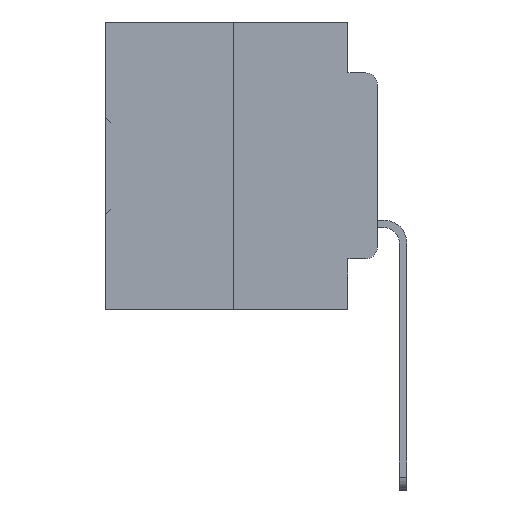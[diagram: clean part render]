
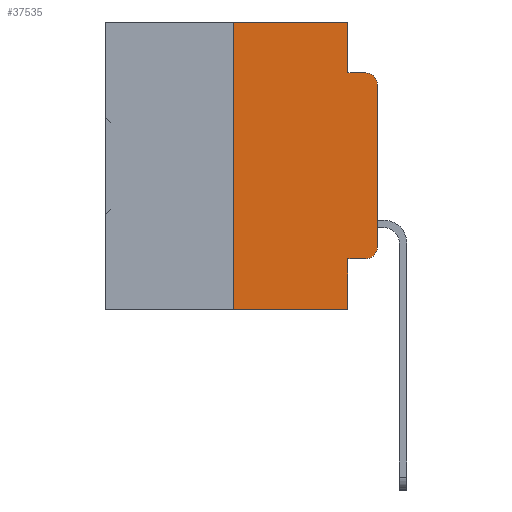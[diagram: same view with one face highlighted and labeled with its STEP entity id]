
A CAD part, left-side view. The second image highlights one B-rep face of the part: STEP entity #37535.
In plain terms, the highlighted planar face has unit normal (-1, 0, 0).
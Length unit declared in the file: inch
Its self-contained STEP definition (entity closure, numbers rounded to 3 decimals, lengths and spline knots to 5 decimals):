
#149 = EDGE_CURVE ( 'NONE', #15255, #26655, #14297, .T. ) ;
#2393 = DIRECTION ( 'NONE',  ( -1., 0., 0. ) ) ;
#2667 = CIRCLE ( 'NONE', #27119, 0.02 ) ;
#3807 = AXIS2_PLACEMENT_3D ( 'NONE', #12877, #33331, #15895 ) ;
#4180 = CARTESIAN_POINT ( 'NONE',  ( 0., 0.051, 0. ) ) ;
#6223 = CARTESIAN_POINT ( 'NONE',  ( 0., 0.051, -0.0885 ) ) ;
#8025 = CARTESIAN_POINT ( 'NONE',  ( 0., 0.25, 0. ) ) ;
#8068 = CARTESIAN_POINT ( 'NONE',  ( 0., 0.02, -0.4115 ) ) ;
#8298 = EDGE_CURVE ( 'NONE', #8849, #34563, #30293, .T. ) ;
#8849 = VERTEX_POINT ( 'NONE', #18146 ) ;
#9312 = LINE ( 'NONE', #22283, #16289 ) ;
#9317 = CARTESIAN_POINT ( 'NONE',  ( 0., 0.25, 0. ) ) ;
#9435 = CARTESIAN_POINT ( 'NONE',  ( 0., 0.02, -0.1085 ) ) ;
#9845 = CARTESIAN_POINT ( 'NONE',  ( 0., 0.02, -0.0885 ) ) ;
#9890 = CARTESIAN_POINT ( 'NONE',  ( 0., 0.051, 0. ) ) ;
#10317 = CARTESIAN_POINT ( 'NONE',  ( 0., 0.051, -0.5 ) ) ;
#11504 = DIRECTION ( 'NONE',  ( 0., -1., 0. ) ) ;
#12415 = DIRECTION ( 'NONE',  ( 0., 0., -1. ) ) ;
#12753 = PLANE ( 'NONE',  #3807 ) ;
#12877 = CARTESIAN_POINT ( 'NONE',  ( 0., 0.473, 0. ) ) ;
#13084 = VECTOR ( 'NONE', #24764, 39.37008 ) ;
#13214 = VERTEX_POINT ( 'NONE', #25533 ) ;
#13695 = EDGE_CURVE ( 'NONE', #14173, #29882, #20017, .T. ) ;
#14173 = VERTEX_POINT ( 'NONE', #8025 ) ;
#14297 = LINE ( 'NONE', #6223, #36649 ) ;
#14536 = ORIENTED_EDGE ( 'NONE', *, *, #15322, .T. ) ;
#14876 = VECTOR ( 'NONE', #24583, 39.37008 ) ;
#15255 = VERTEX_POINT ( 'NONE', #24947 ) ;
#15322 = EDGE_CURVE ( 'NONE', #20189, #30032, #9312, .T. ) ;
#15479 = CARTESIAN_POINT ( 'NONE',  ( 0., 0.051, 0. ) ) ;
#15895 = DIRECTION ( 'NONE',  ( 0., 0., -1. ) ) ;
#15964 = ORIENTED_EDGE ( 'NONE', *, *, #31698, .T. ) ;
#16280 = EDGE_CURVE ( 'NONE', #13214, #14173, #26963, .T. ) ;
#16289 = VECTOR ( 'NONE', #16528, 39.37008 ) ;
#16528 = DIRECTION ( 'NONE',  ( 0., 0., 1. ) ) ;
#16646 = CARTESIAN_POINT ( 'NONE',  ( 0., 0., -0.1085 ) ) ;
#16747 = ORIENTED_EDGE ( 'NONE', *, *, #149, .F. ) ;
#16749 = LINE ( 'NONE', #9890, #14876 ) ;
#17226 = ORIENTED_EDGE ( 'NONE', *, *, #26038, .F. ) ;
#17313 = CARTESIAN_POINT ( 'NONE',  ( 0., 0.051, -0.4115 ) ) ;
#18146 = CARTESIAN_POINT ( 'NONE',  ( 0., 0.051, -0.4115 ) ) ;
#18939 = ORIENTED_EDGE ( 'NONE', *, *, #13695, .F. ) ;
#19048 = VECTOR ( 'NONE', #11504, 39.37008 ) ;
#19998 = ORIENTED_EDGE ( 'NONE', *, *, #16280, .F. ) ;
#20017 = LINE ( 'NONE', #21830, #13084 ) ;
#20113 = CARTESIAN_POINT ( 'NONE',  ( 0., 0.02, -0.3915 ) ) ;
#20189 = VERTEX_POINT ( 'NONE', #36355 ) ;
#20435 = CIRCLE ( 'NONE', #23764, 0.02 ) ;
#21830 = CARTESIAN_POINT ( 'NONE',  ( 0., 0.473, 0. ) ) ;
#21871 = ORIENTED_EDGE ( 'NONE', *, *, #29089, .T. ) ;
#22082 = FACE_OUTER_BOUND ( 'NONE', #23550, .T. ) ;
#22283 = CARTESIAN_POINT ( 'NONE',  ( 0., 0., 0. ) ) ;
#22598 = VECTOR ( 'NONE', #24304, 39.37008 ) ;
#22808 = ORIENTED_EDGE ( 'NONE', *, *, #8298, .F. ) ;
#23064 = DIRECTION ( 'NONE',  ( 0., 0., -1. ) ) ;
#23550 = EDGE_LOOP ( 'NONE', ( #14536, #15964, #16747, #17226, #18939, #19998, #21871, #22808, #24181, #25751 ) ) ;
#23764 = AXIS2_PLACEMENT_3D ( 'NONE', #20113, #2393, #23064 ) ;
#24181 = ORIENTED_EDGE ( 'NONE', *, *, #36495, .T. ) ;
#24304 = DIRECTION ( 'NONE',  ( 0., 0., -1. ) ) ;
#24583 = DIRECTION ( 'NONE',  ( 0., 0., -1. ) ) ;
#24764 = DIRECTION ( 'NONE',  ( 0., -1., 0. ) ) ;
#24831 = EDGE_CURVE ( 'NONE', #37793, #20189, #20435, .T. ) ;
#24947 = CARTESIAN_POINT ( 'NONE',  ( 0., 0.051, -0.0885 ) ) ;
#25533 = CARTESIAN_POINT ( 'NONE',  ( 0., 0.25, -0.5 ) ) ;
#25751 = ORIENTED_EDGE ( 'NONE', *, *, #24831, .T. ) ;
#25865 = LINE ( 'NONE', #26127, #19048 ) ;
#26038 = EDGE_CURVE ( 'NONE', #29882, #15255, #16749, .T. ) ;
#26127 = CARTESIAN_POINT ( 'NONE',  ( 0., 0.473, -0.5 ) ) ;
#26655 = VERTEX_POINT ( 'NONE', #9845 ) ;
#26932 = DIRECTION ( 'NONE',  ( 0., 0., 1. ) ) ;
#26963 = LINE ( 'NONE', #9317, #33770 ) ;
#27119 = AXIS2_PLACEMENT_3D ( 'NONE', #9435, #29958, #12415 ) ;
#27896 = LINE ( 'NONE', #17313, #30339 ) ;
#29089 = EDGE_CURVE ( 'NONE', #13214, #34563, #25865, .T. ) ;
#29518 = DIRECTION ( 'NONE',  ( 0., -1., 0. ) ) ;
#29882 = VERTEX_POINT ( 'NONE', #4180 ) ;
#29958 = DIRECTION ( 'NONE',  ( -1., 0., 0. ) ) ;
#30032 = VERTEX_POINT ( 'NONE', #16646 ) ;
#30293 = LINE ( 'NONE', #15479, #22598 ) ;
#30339 = VECTOR ( 'NONE', #31821, 39.37008 ) ;
#31698 = EDGE_CURVE ( 'NONE', #30032, #26655, #2667, .T. ) ;
#31821 = DIRECTION ( 'NONE',  ( 0., -1., 0. ) ) ;
#33331 = DIRECTION ( 'NONE',  ( 1., 0., 0. ) ) ;
#33770 = VECTOR ( 'NONE', #26932, 39.37008 ) ;
#34563 = VERTEX_POINT ( 'NONE', #10317 ) ;
#36355 = CARTESIAN_POINT ( 'NONE',  ( 0., 0., -0.3915 ) ) ;
#36495 = EDGE_CURVE ( 'NONE', #8849, #37793, #27896, .T. ) ;
#36649 = VECTOR ( 'NONE', #29518, 39.37008 ) ;
#37535 = ADVANCED_FACE ( 'NONE', ( #22082 ), #12753, .F. ) ;
#37793 = VERTEX_POINT ( 'NONE', #8068 ) ;
